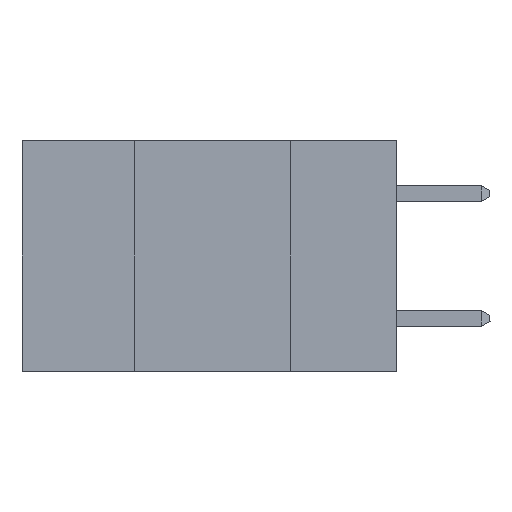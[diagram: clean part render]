
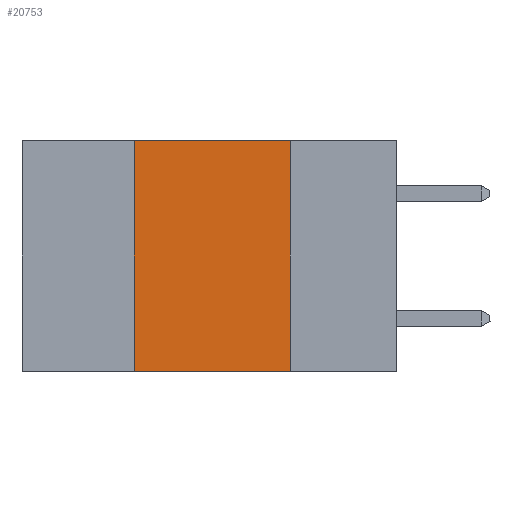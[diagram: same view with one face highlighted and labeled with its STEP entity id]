
A CAD part, left-side view. The second image highlights one B-rep face of the part: STEP entity #20753.
In plain terms, the highlighted planar face has unit normal (-1, 0, 0).
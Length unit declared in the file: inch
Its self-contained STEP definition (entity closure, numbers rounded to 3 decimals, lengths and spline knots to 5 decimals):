
#653 = LINE ( 'NONE', #5710, #22218 ) ;
#1339 = CARTESIAN_POINT ( 'NONE',  ( 0., 0.42, 0. ) ) ;
#2417 = FACE_OUTER_BOUND ( 'NONE', #24504, .T. ) ;
#2434 = ORIENTED_EDGE ( 'NONE', *, *, #13535, .F. ) ;
#2744 = DIRECTION ( 'NONE',  ( 0., -1., 0. ) ) ;
#2810 = VERTEX_POINT ( 'NONE', #24802 ) ;
#4633 = VERTEX_POINT ( 'NONE', #14829 ) ;
#5323 = EDGE_CURVE ( 'NONE', #2810, #14258, #11023, .T. ) ;
#5710 = CARTESIAN_POINT ( 'NONE',  ( 0., 0.6, -0.37 ) ) ;
#5869 = ORIENTED_EDGE ( 'NONE', *, *, #18884, .F. ) ;
#5937 = LINE ( 'NONE', #1339, #21422 ) ;
#6081 = DIRECTION ( 'NONE',  ( 0., 0., -1. ) ) ;
#10045 = PLANE ( 'NONE',  #23625 ) ;
#10947 = DIRECTION ( 'NONE',  ( 0., 0., -1. ) ) ;
#11023 = LINE ( 'NONE', #21035, #21686 ) ;
#12148 = CARTESIAN_POINT ( 'NONE',  ( 0., 0.6, 0. ) ) ;
#13535 = EDGE_CURVE ( 'NONE', #18437, #4633, #5937, .T. ) ;
#13656 = CARTESIAN_POINT ( 'NONE',  ( 0., 0.42, -0.37 ) ) ;
#13865 = ORIENTED_EDGE ( 'NONE', *, *, #16573, .T. ) ;
#14023 = ORIENTED_EDGE ( 'NONE', *, *, #5323, .F. ) ;
#14258 = VERTEX_POINT ( 'NONE', #17842 ) ;
#14829 = CARTESIAN_POINT ( 'NONE',  ( 0., 0.42, 0. ) ) ;
#16573 = EDGE_CURVE ( 'NONE', #18437, #14258, #653, .T. ) ;
#16974 = CARTESIAN_POINT ( 'NONE',  ( 0., 0.6, 0. ) ) ;
#17842 = CARTESIAN_POINT ( 'NONE',  ( 0., 0.17, -0.37 ) ) ;
#18190 = DIRECTION ( 'NONE',  ( 1., 0., 0. ) ) ;
#18437 = VERTEX_POINT ( 'NONE', #13656 ) ;
#18884 = EDGE_CURVE ( 'NONE', #4633, #2810, #25180, .T. ) ;
#19867 = DIRECTION ( 'NONE',  ( 0., -1., 0. ) ) ;
#20753 = ADVANCED_FACE ( 'NONE', ( #2417 ), #10045, .F. ) ;
#21035 = CARTESIAN_POINT ( 'NONE',  ( 0., 0.17, 0. ) ) ;
#21422 = VECTOR ( 'NONE', #25618, 39.37008 ) ;
#21686 = VECTOR ( 'NONE', #10947, 39.37008 ) ;
#22218 = VECTOR ( 'NONE', #19867, 39.37008 ) ;
#23625 = AXIS2_PLACEMENT_3D ( 'NONE', #12148, #18190, #6081 ) ;
#24504 = EDGE_LOOP ( 'NONE', ( #14023, #5869, #2434, #13865 ) ) ;
#24802 = CARTESIAN_POINT ( 'NONE',  ( 0., 0.17, 0. ) ) ;
#25180 = LINE ( 'NONE', #16974, #25808 ) ;
#25618 = DIRECTION ( 'NONE',  ( 0., 0., 1. ) ) ;
#25808 = VECTOR ( 'NONE', #2744, 39.37008 ) ;
